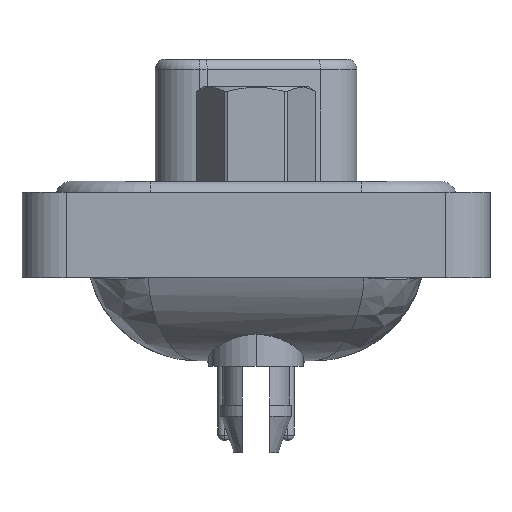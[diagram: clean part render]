
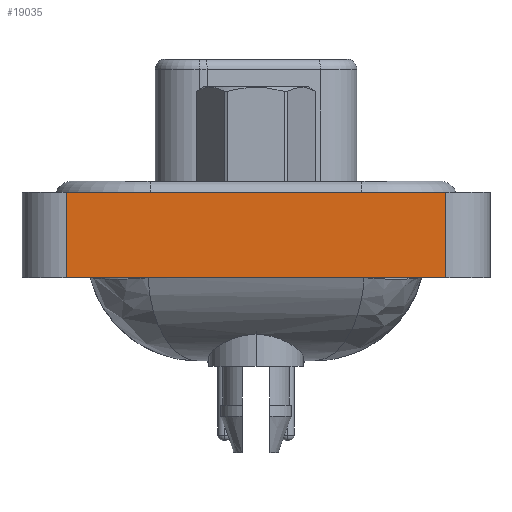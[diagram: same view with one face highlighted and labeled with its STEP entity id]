
A CAD part, left-side view. The second image highlights one B-rep face of the part: STEP entity #19035.
In plain terms, the highlighted planar face has unit normal (-1, 0, 0).
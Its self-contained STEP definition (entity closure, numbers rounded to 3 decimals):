
#1520 = VERTEX_POINT ( 'NONE', #15211 ) ;
#1543 = CARTESIAN_POINT ( 'NONE',  ( -7.25, 8.55, -3.35 ) ) ;
#1623 = VECTOR ( 'NONE', #3149, 1000. ) ;
#2335 = ORIENTED_EDGE ( 'NONE', *, *, #20036, .F. ) ;
#2605 = VECTOR ( 'NONE', #8469, 1000. ) ;
#3149 = DIRECTION ( 'NONE',  ( 0., 0., 1. ) ) ;
#3868 = VERTEX_POINT ( 'NONE', #13350 ) ;
#4194 = PLANE ( 'NONE',  #7965 ) ;
#5481 = DIRECTION ( 'NONE',  ( 0., 0., 1. ) ) ;
#6422 = LINE ( 'NONE', #8416, #1623 ) ;
#7050 = CARTESIAN_POINT ( 'NONE',  ( -7.25, -8.55, -3.35 ) ) ;
#7965 = AXIS2_PLACEMENT_3D ( 'NONE', #13816, #18260, #5481 ) ;
#8284 = VECTOR ( 'NONE', #14943, 1000. ) ;
#8416 = CARTESIAN_POINT ( 'NONE',  ( -7.25, 8.55, -3.35 ) ) ;
#8469 = DIRECTION ( 'NONE',  ( 0., 0., 1. ) ) ;
#9232 = CARTESIAN_POINT ( 'NONE',  ( -7.25, 8.55, 0.5 ) ) ;
#9978 = EDGE_CURVE ( 'NONE', #19373, #3868, #13608, .T. ) ;
#11041 = ORIENTED_EDGE ( 'NONE', *, *, #12453, .T. ) ;
#11661 = LINE ( 'NONE', #11773, #8284 ) ;
#11773 = CARTESIAN_POINT ( 'NONE',  ( -7.25, -8.55, 0.5 ) ) ;
#11846 = VECTOR ( 'NONE', #16674, 1000. ) ;
#12039 = FACE_OUTER_BOUND ( 'NONE', #14590, .T. ) ;
#12453 = EDGE_CURVE ( 'NONE', #3868, #1520, #13230, .T. ) ;
#12737 = ORIENTED_EDGE ( 'NONE', *, *, #9978, .T. ) ;
#13230 = LINE ( 'NONE', #19761, #2605 ) ;
#13350 = CARTESIAN_POINT ( 'NONE',  ( -7.25, -8.55, -3.35 ) ) ;
#13608 = LINE ( 'NONE', #7050, #11846 ) ;
#13816 = CARTESIAN_POINT ( 'NONE',  ( -7.25, -8.55, -3.35 ) ) ;
#14590 = EDGE_LOOP ( 'NONE', ( #11041, #2335, #17022, #12737 ) ) ;
#14943 = DIRECTION ( 'NONE',  ( 0., -1., 0. ) ) ;
#15131 = VERTEX_POINT ( 'NONE', #9232 ) ;
#15211 = CARTESIAN_POINT ( 'NONE',  ( -7.25, -8.55, 0.5 ) ) ;
#15554 = EDGE_CURVE ( 'NONE', #19373, #15131, #6422, .T. ) ;
#16674 = DIRECTION ( 'NONE',  ( 0., -1., 0. ) ) ;
#17022 = ORIENTED_EDGE ( 'NONE', *, *, #15554, .F. ) ;
#18260 = DIRECTION ( 'NONE',  ( -1., 0., 0. ) ) ;
#19035 = ADVANCED_FACE ( 'NONE', ( #12039 ), #4194, .T. ) ;
#19373 = VERTEX_POINT ( 'NONE', #1543 ) ;
#19761 = CARTESIAN_POINT ( 'NONE',  ( -7.25, -8.55, -3.35 ) ) ;
#20036 = EDGE_CURVE ( 'NONE', #15131, #1520, #11661, .T. ) ;
